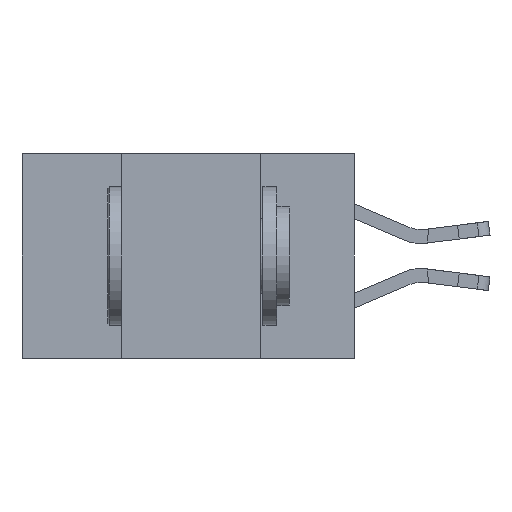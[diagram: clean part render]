
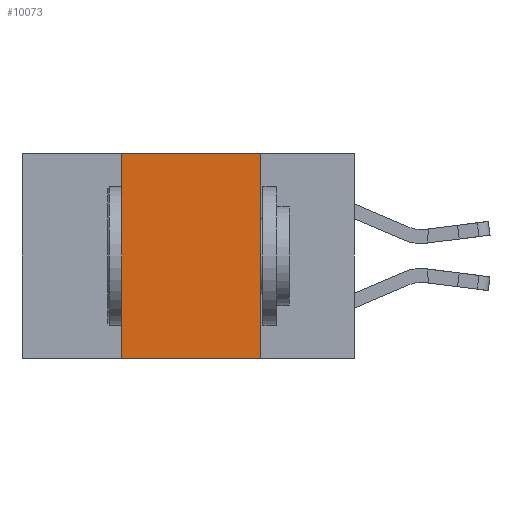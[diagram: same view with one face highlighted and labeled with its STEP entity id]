
A CAD part, left-side view. The second image highlights one B-rep face of the part: STEP entity #10073.
In plain terms, the highlighted planar face has unit normal (-1, 0, 0).
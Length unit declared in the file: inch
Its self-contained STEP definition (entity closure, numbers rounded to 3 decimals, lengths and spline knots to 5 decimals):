
#441 = CARTESIAN_POINT ( 'NONE',  ( 0., 0.6, 0. ) ) ;
#502 = VERTEX_POINT ( 'NONE', #8303 ) ;
#2115 = LINE ( 'NONE', #13592, #4781 ) ;
#3239 = CARTESIAN_POINT ( 'NONE',  ( 0., 0.42, -0.37 ) ) ;
#3840 = LINE ( 'NONE', #15504, #10131 ) ;
#4681 = DIRECTION ( 'NONE',  ( 0., 0., -1. ) ) ;
#4781 = VECTOR ( 'NONE', #17251, 39.37008 ) ;
#4803 = FACE_OUTER_BOUND ( 'NONE', #17552, .T. ) ;
#5329 = CARTESIAN_POINT ( 'NONE',  ( 0., 0.17, -0.37 ) ) ;
#5444 = LINE ( 'NONE', #5329, #19611 ) ;
#6094 = CARTESIAN_POINT ( 'NONE',  ( 0., 0.17, 0. ) ) ;
#6395 = VERTEX_POINT ( 'NONE', #3239 ) ;
#6467 = EDGE_CURVE ( 'NONE', #20157, #19482, #12698, .T. ) ;
#6814 = EDGE_CURVE ( 'NONE', #6395, #502, #3840, .T. ) ;
#8303 = CARTESIAN_POINT ( 'NONE',  ( 0., 0.17, -0.37 ) ) ;
#8371 = CARTESIAN_POINT ( 'NONE',  ( 0., 0.6, 0. ) ) ;
#8692 = AXIS2_PLACEMENT_3D ( 'NONE', #8371, #18366, #4681 ) ;
#9042 = DIRECTION ( 'NONE',  ( 0., -1., 0. ) ) ;
#9799 = CARTESIAN_POINT ( 'NONE',  ( 0., 0.42, 0. ) ) ;
#10073 = ADVANCED_FACE ( 'NONE', ( #4803 ), #16902, .F. ) ;
#10131 = VECTOR ( 'NONE', #10189, 39.37008 ) ;
#10189 = DIRECTION ( 'NONE',  ( 0., -1., 0. ) ) ;
#12216 = DIRECTION ( 'NONE',  ( 0., 0., -1. ) ) ;
#12698 = LINE ( 'NONE', #441, #12959 ) ;
#12959 = VECTOR ( 'NONE', #9042, 39.37008 ) ;
#13351 = ORIENTED_EDGE ( 'NONE', *, *, #19832, .F. ) ;
#13592 = CARTESIAN_POINT ( 'NONE',  ( 0., 0.42, -0.37 ) ) ;
#15504 = CARTESIAN_POINT ( 'NONE',  ( 0., 0.6, -0.37 ) ) ;
#16902 = PLANE ( 'NONE',  #8692 ) ;
#17251 = DIRECTION ( 'NONE',  ( 0., 0., 1. ) ) ;
#17552 = EDGE_LOOP ( 'NONE', ( #21625, #18112, #13351, #18285 ) ) ;
#17799 = EDGE_CURVE ( 'NONE', #19482, #502, #5444, .T. ) ;
#18112 = ORIENTED_EDGE ( 'NONE', *, *, #6467, .F. ) ;
#18285 = ORIENTED_EDGE ( 'NONE', *, *, #6814, .T. ) ;
#18366 = DIRECTION ( 'NONE',  ( 1., 0., 0. ) ) ;
#19482 = VERTEX_POINT ( 'NONE', #6094 ) ;
#19611 = VECTOR ( 'NONE', #12216, 39.37008 ) ;
#19832 = EDGE_CURVE ( 'NONE', #6395, #20157, #2115, .T. ) ;
#20157 = VERTEX_POINT ( 'NONE', #9799 ) ;
#21625 = ORIENTED_EDGE ( 'NONE', *, *, #17799, .F. ) ;
